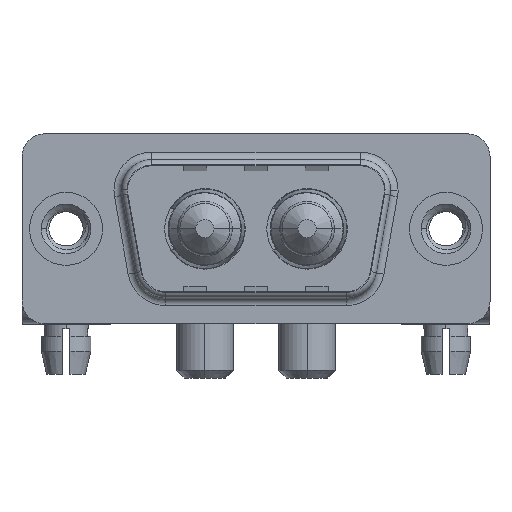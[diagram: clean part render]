
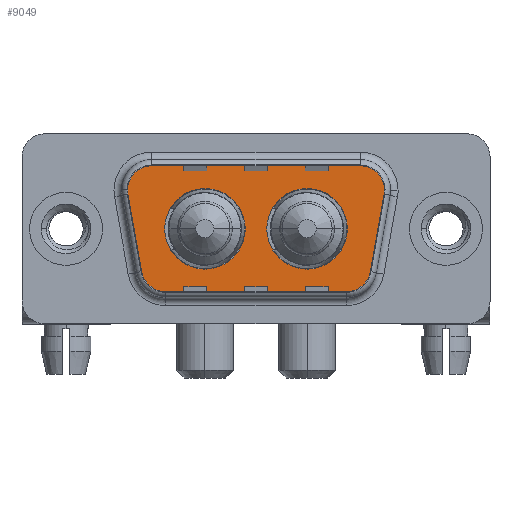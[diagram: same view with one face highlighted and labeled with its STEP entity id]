
A CAD part, top view. The second image highlights one B-rep face of the part: STEP entity #9049.
In plain terms, the highlighted planar face has unit normal (0, 0, 1).
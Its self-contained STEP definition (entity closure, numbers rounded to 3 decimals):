
#69 = ORIENTED_EDGE ( 'NONE', *, *, #13640, .T. ) ;
#169 = AXIS2_PLACEMENT_3D ( 'NONE', #11451, #8176, #579 ) ;
#422 = VECTOR ( 'NONE', #12677, 1000. ) ;
#488 = VERTEX_POINT ( 'NONE', #3157 ) ;
#531 = CARTESIAN_POINT ( 'NONE',  ( 6.459, -4.9, 0. ) ) ;
#579 = DIRECTION ( 'NONE',  ( -1., 0., 0. ) ) ;
#596 = CARTESIAN_POINT ( 'NONE',  ( 9.14, 0., 0. ) ) ;
#599 = FACE_BOUND ( 'NONE', #9286, .T. ) ;
#686 = ORIENTED_EDGE ( 'NONE', *, *, #7650, .F. ) ;
#745 = AXIS2_PLACEMENT_3D ( 'NONE', #1173, #13953, #2038 ) ;
#834 = AXIS2_PLACEMENT_3D ( 'NONE', #2820, #7186, #11538 ) ;
#1060 = DIRECTION ( 'NONE',  ( 0., 0., 1. ) ) ;
#1064 = CARTESIAN_POINT ( 'NONE',  ( 13.21, 0., 0. ) ) ;
#1145 = DIRECTION ( 'NONE',  ( 0., 0., 1. ) ) ;
#1173 = CARTESIAN_POINT ( 'NONE',  ( 19.564, 2.9, 0. ) ) ;
#1283 = CARTESIAN_POINT ( 'NONE',  ( 5.436, 2.9, 0. ) ) ;
#1284 = LINE ( 'NONE', #5001, #14061 ) ;
#1542 = AXIS2_PLACEMENT_3D ( 'NONE', #4816, #9168, #13801 ) ;
#1769 = EDGE_CURVE ( 'NONE', #7991, #2988, #7024, .T. ) ;
#1895 = CIRCLE ( 'NONE', #7149, 2.65 ) ;
#2038 = DIRECTION ( 'NONE',  ( -1., 0., 0. ) ) ;
#2369 = EDGE_CURVE ( 'NONE', #13620, #11448, #12505, .T. ) ;
#2634 = LINE ( 'NONE', #13555, #7248 ) ;
#2793 = AXIS2_PLACEMENT_3D ( 'NONE', #1283, #1145, #11985 ) ;
#2820 = CARTESIAN_POINT ( 'NONE',  ( 18.541, -2.9, 0. ) ) ;
#2975 = ORIENTED_EDGE ( 'NONE', *, *, #6294, .T. ) ;
#2988 = VERTEX_POINT ( 'NONE', #13491 ) ;
#2998 = CARTESIAN_POINT ( 'NONE',  ( 5.436, 4.9, 0. ) ) ;
#3157 = CARTESIAN_POINT ( 'NONE',  ( 4.489, -3.247, 0. ) ) ;
#3200 = VERTEX_POINT ( 'NONE', #6340 ) ;
#3294 = EDGE_CURVE ( 'NONE', #9255, #7368, #1895, .T. ) ;
#3312 = EDGE_CURVE ( 'NONE', #8254, #7991, #11470, .T. ) ;
#3813 = EDGE_LOOP ( 'NONE', ( #12979, #8665, #2975, #12491, #12776, #69, #4894, #8944, #6197 ) ) ;
#3925 = DIRECTION ( 'NONE',  ( 0.174, 0.985, 0. ) ) ;
#4018 = DIRECTION ( 'NONE',  ( 0., 0., 1. ) ) ;
#4162 = CARTESIAN_POINT ( 'NONE',  ( 6.459, -4.9, 0. ) ) ;
#4214 = CARTESIAN_POINT ( 'NONE',  ( 15.86, 0., 0. ) ) ;
#4531 = CARTESIAN_POINT ( 'NONE',  ( 18.51, 0., 0. ) ) ;
#4648 = CIRCLE ( 'NONE', #745, 2. ) ;
#4776 = DIRECTION ( 'NONE',  ( 0., 0., 1. ) ) ;
#4816 = CARTESIAN_POINT ( 'NONE',  ( 15.86, 0., 0. ) ) ;
#4894 = ORIENTED_EDGE ( 'NONE', *, *, #6708, .T. ) ;
#4931 = ORIENTED_EDGE ( 'NONE', *, *, #2369, .F. ) ;
#4980 = FACE_OUTER_BOUND ( 'NONE', #3813, .T. ) ;
#4985 = CARTESIAN_POINT ( 'NONE',  ( 9.14, 0., 0. ) ) ;
#5001 = CARTESIAN_POINT ( 'NONE',  ( 21.534, 2.553, 0. ) ) ;
#5652 = CIRCLE ( 'NONE', #1542, 2.65 ) ;
#6103 = LINE ( 'NONE', #8329, #422 ) ;
#6105 = AXIS2_PLACEMENT_3D ( 'NONE', #10711, #9626, #8358 ) ;
#6197 = ORIENTED_EDGE ( 'NONE', *, *, #3312, .T. ) ;
#6294 = EDGE_CURVE ( 'NONE', #12442, #3200, #12265, .T. ) ;
#6340 = CARTESIAN_POINT ( 'NONE',  ( 21.564, 2.9, 0. ) ) ;
#6708 = EDGE_CURVE ( 'NONE', #11806, #488, #2634, .T. ) ;
#7024 = CIRCLE ( 'NONE', #13857, 2. ) ;
#7149 = AXIS2_PLACEMENT_3D ( 'NONE', #4985, #4776, #13473 ) ;
#7186 = DIRECTION ( 'NONE',  ( 0., 0., 1. ) ) ;
#7248 = VECTOR ( 'NONE', #11206, 1000. ) ;
#7368 = VERTEX_POINT ( 'NONE', #8841 ) ;
#7650 = EDGE_CURVE ( 'NONE', #7368, #9255, #8881, .T. ) ;
#7667 = EDGE_CURVE ( 'NONE', #12043, #10642, #6103, .T. ) ;
#7991 = VERTEX_POINT ( 'NONE', #13517 ) ;
#8176 = DIRECTION ( 'NONE',  ( 0., 0., 1. ) ) ;
#8239 = ORIENTED_EDGE ( 'NONE', *, *, #9446, .F. ) ;
#8254 = VERTEX_POINT ( 'NONE', #4162 ) ;
#8259 = DIRECTION ( 'NONE',  ( 0., 0., 1. ) ) ;
#8329 = CARTESIAN_POINT ( 'NONE',  ( 5.436, 4.9, 0. ) ) ;
#8358 = DIRECTION ( 'NONE',  ( -1., 0., 0. ) ) ;
#8418 = EDGE_CURVE ( 'NONE', #2988, #12442, #1284, .T. ) ;
#8665 = ORIENTED_EDGE ( 'NONE', *, *, #8418, .T. ) ;
#8841 = CARTESIAN_POINT ( 'NONE',  ( 11.79, 0., 0. ) ) ;
#8881 = CIRCLE ( 'NONE', #9098, 2.65 ) ;
#8944 = ORIENTED_EDGE ( 'NONE', *, *, #9443, .T. ) ;
#8980 = VECTOR ( 'NONE', #9123, 1000. ) ;
#9049 = ADVANCED_FACE ( 'NONE', ( #9185, #599, #4980 ), #13819, .T. ) ;
#9098 = AXIS2_PLACEMENT_3D ( 'NONE', #596, #8259, #11536 ) ;
#9123 = DIRECTION ( 'NONE',  ( 1., 0., 0. ) ) ;
#9168 = DIRECTION ( 'NONE',  ( 0., 0., 1. ) ) ;
#9185 = FACE_BOUND ( 'NONE', #12338, .T. ) ;
#9255 = VERTEX_POINT ( 'NONE', #13456 ) ;
#9286 = EDGE_LOOP ( 'NONE', ( #686, #11083 ) ) ;
#9443 = EDGE_CURVE ( 'NONE', #488, #8254, #14085, .T. ) ;
#9446 = EDGE_CURVE ( 'NONE', #11448, #13620, #5652, .T. ) ;
#9626 = DIRECTION ( 'NONE',  ( 0., 0., 1. ) ) ;
#10456 = CARTESIAN_POINT ( 'NONE',  ( 21.534, 2.553, 0. ) ) ;
#10575 = DIRECTION ( 'NONE',  ( 1., 0., 0. ) ) ;
#10642 = VERTEX_POINT ( 'NONE', #2998 ) ;
#10711 = CARTESIAN_POINT ( 'NONE',  ( 19.564, 2.9, 0. ) ) ;
#11061 = CARTESIAN_POINT ( 'NONE',  ( 3.466, 2.553, 0. ) ) ;
#11083 = ORIENTED_EDGE ( 'NONE', *, *, #3294, .F. ) ;
#11206 = DIRECTION ( 'NONE',  ( 0.174, -0.985, 0. ) ) ;
#11448 = VERTEX_POINT ( 'NONE', #4531 ) ;
#11451 = CARTESIAN_POINT ( 'NONE',  ( 6.459, -2.9, 0. ) ) ;
#11470 = LINE ( 'NONE', #531, #8980 ) ;
#11536 = DIRECTION ( 'NONE',  ( 1., 0., 0. ) ) ;
#11538 = DIRECTION ( 'NONE',  ( 1., 0., 0. ) ) ;
#11806 = VERTEX_POINT ( 'NONE', #11061 ) ;
#11985 = DIRECTION ( 'NONE',  ( 1., 0., 0. ) ) ;
#12043 = VERTEX_POINT ( 'NONE', #13830 ) ;
#12265 = CIRCLE ( 'NONE', #6105, 2. ) ;
#12338 = EDGE_LOOP ( 'NONE', ( #8239, #4931 ) ) ;
#12442 = VERTEX_POINT ( 'NONE', #10456 ) ;
#12491 = ORIENTED_EDGE ( 'NONE', *, *, #14064, .T. ) ;
#12505 = CIRCLE ( 'NONE', #13422, 2.65 ) ;
#12516 = CARTESIAN_POINT ( 'NONE',  ( 18.541, -2.9, 0. ) ) ;
#12677 = DIRECTION ( 'NONE',  ( -1., 0., 0. ) ) ;
#12776 = ORIENTED_EDGE ( 'NONE', *, *, #7667, .T. ) ;
#12830 = CIRCLE ( 'NONE', #2793, 2. ) ;
#12979 = ORIENTED_EDGE ( 'NONE', *, *, #1769, .T. ) ;
#13422 = AXIS2_PLACEMENT_3D ( 'NONE', #4214, #1060, #13919 ) ;
#13456 = CARTESIAN_POINT ( 'NONE',  ( 6.49, 0., 0. ) ) ;
#13473 = DIRECTION ( 'NONE',  ( 1., 0., 0. ) ) ;
#13491 = CARTESIAN_POINT ( 'NONE',  ( 20.511, -3.247, 0. ) ) ;
#13517 = CARTESIAN_POINT ( 'NONE',  ( 18.541, -4.9, 0. ) ) ;
#13555 = CARTESIAN_POINT ( 'NONE',  ( 3.466, 2.553, 0. ) ) ;
#13620 = VERTEX_POINT ( 'NONE', #1064 ) ;
#13640 = EDGE_CURVE ( 'NONE', #10642, #11806, #12830, .T. ) ;
#13801 = DIRECTION ( 'NONE',  ( 1., 0., 0. ) ) ;
#13819 = PLANE ( 'NONE',  #834 ) ;
#13830 = CARTESIAN_POINT ( 'NONE',  ( 19.564, 4.9, 0. ) ) ;
#13857 = AXIS2_PLACEMENT_3D ( 'NONE', #12516, #4018, #10575 ) ;
#13919 = DIRECTION ( 'NONE',  ( 1., 0., 0. ) ) ;
#13953 = DIRECTION ( 'NONE',  ( 0., 0., 1. ) ) ;
#14061 = VECTOR ( 'NONE', #3925, 1000. ) ;
#14064 = EDGE_CURVE ( 'NONE', #3200, #12043, #4648, .T. ) ;
#14085 = CIRCLE ( 'NONE', #169, 2. ) ;
